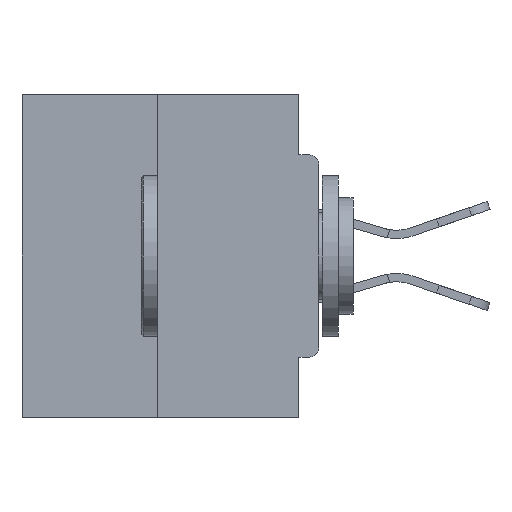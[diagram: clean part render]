
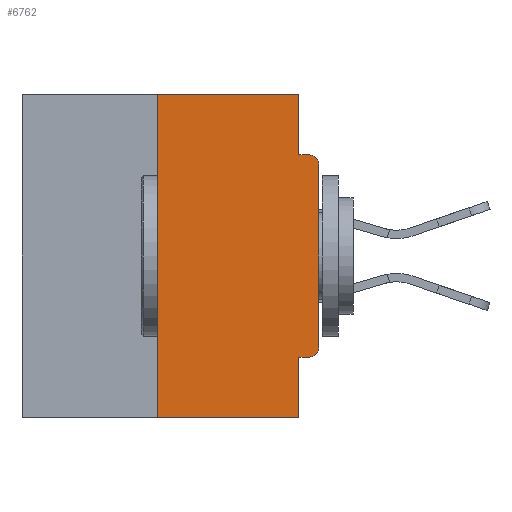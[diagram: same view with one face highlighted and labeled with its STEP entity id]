
A CAD part, left-side view. The second image highlights one B-rep face of the part: STEP entity #6762.
In plain terms, the highlighted planar face has unit normal (-1, 0, 0).
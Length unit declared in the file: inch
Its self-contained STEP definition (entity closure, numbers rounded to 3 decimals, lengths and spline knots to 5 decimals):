
#129 = VERTEX_POINT ( 'NONE', #37225 ) ;
#652 = LINE ( 'NONE', #36962, #32376 ) ;
#769 = ORIENTED_EDGE ( 'NONE', *, *, #18249, .F. ) ;
#838 = DIRECTION ( 'NONE',  ( -1., 0., 0. ) ) ;
#1036 = EDGE_LOOP ( 'NONE', ( #4687, #27229, #32457, #11501, #16882, #5489, #13640, #4862, #15352, #769 ) ) ;
#1515 = EDGE_CURVE ( 'NONE', #34537, #17718, #652, .T. ) ;
#1567 = EDGE_CURVE ( 'NONE', #35840, #129, #34365, .T. ) ;
#3018 = VERTEX_POINT ( 'NONE', #20286 ) ;
#3319 = VERTEX_POINT ( 'NONE', #10467 ) ;
#4687 = ORIENTED_EDGE ( 'NONE', *, *, #25643, .F. ) ;
#4862 = ORIENTED_EDGE ( 'NONE', *, *, #39757, .T. ) ;
#5489 = ORIENTED_EDGE ( 'NONE', *, *, #23468, .T. ) ;
#6762 = ADVANCED_FACE ( 'NONE', ( #23129 ), #31804, .F. ) ;
#7204 = DIRECTION ( 'NONE',  ( 0., 0., -1. ) ) ;
#7487 = LINE ( 'NONE', #32977, #12406 ) ;
#8278 = AXIS2_PLACEMENT_3D ( 'NONE', #34851, #838, #7204 ) ;
#8738 = CARTESIAN_POINT ( 'NONE',  ( 0., 0.031, -0.5 ) ) ;
#8746 = VECTOR ( 'NONE', #33894, 39.37008 ) ;
#9905 = VECTOR ( 'NONE', #30949, 39.37008 ) ;
#10383 = LINE ( 'NONE', #31105, #28981 ) ;
#10467 = CARTESIAN_POINT ( 'NONE',  ( 0., 0.25, -0.5 ) ) ;
#10676 = VERTEX_POINT ( 'NONE', #13329 ) ;
#11501 = ORIENTED_EDGE ( 'NONE', *, *, #18194, .F. ) ;
#11875 = DIRECTION ( 'NONE',  ( 0., 0., -1. ) ) ;
#12406 = VECTOR ( 'NONE', #39248, 39.37008 ) ;
#12536 = DIRECTION ( 'NONE',  ( 0., 0., 1. ) ) ;
#13329 = CARTESIAN_POINT ( 'NONE',  ( 0., 0.031, 0. ) ) ;
#13640 = ORIENTED_EDGE ( 'NONE', *, *, #1567, .T. ) ;
#13912 = EDGE_CURVE ( 'NONE', #3319, #16950, #10383, .T. ) ;
#15352 = ORIENTED_EDGE ( 'NONE', *, *, #1515, .F. ) ;
#15774 = CARTESIAN_POINT ( 'NONE',  ( 0., 0., -0.4065 ) ) ;
#16099 = VECTOR ( 'NONE', #11875, 39.37008 ) ;
#16106 = CARTESIAN_POINT ( 'NONE',  ( 0., 0.46, 0. ) ) ;
#16556 = DIRECTION ( 'NONE',  ( 0., 0., -1. ) ) ;
#16637 = DIRECTION ( 'NONE',  ( 1., 0., 0. ) ) ;
#16882 = ORIENTED_EDGE ( 'NONE', *, *, #21723, .F. ) ;
#16950 = VERTEX_POINT ( 'NONE', #20028 ) ;
#17718 = VERTEX_POINT ( 'NONE', #20878 ) ;
#17770 = CARTESIAN_POINT ( 'NONE',  ( 0., 0.031, -0.4065 ) ) ;
#18194 = EDGE_CURVE ( 'NONE', #32849, #3018, #19501, .T. ) ;
#18249 = EDGE_CURVE ( 'NONE', #10676, #34537, #26800, .T. ) ;
#19450 = CIRCLE ( 'NONE', #30038, 0.015 ) ;
#19501 = LINE ( 'NONE', #8738, #16099 ) ;
#19564 = CARTESIAN_POINT ( 'NONE',  ( 0., 0.015, -0.3915 ) ) ;
#19647 = DIRECTION ( 'NONE',  ( 0., 0., -1. ) ) ;
#20028 = CARTESIAN_POINT ( 'NONE',  ( 0., 0.25, 0. ) ) ;
#20216 = LINE ( 'NONE', #15774, #35386 ) ;
#20286 = CARTESIAN_POINT ( 'NONE',  ( 0., 0.031, -0.5 ) ) ;
#20372 = VECTOR ( 'NONE', #27808, 39.37008 ) ;
#20878 = CARTESIAN_POINT ( 'NONE',  ( 0., 0.015, -0.0935 ) ) ;
#21340 = CARTESIAN_POINT ( 'NONE',  ( 0., 0.031, 0. ) ) ;
#21580 = CARTESIAN_POINT ( 'NONE',  ( 0., 0., -0.3915 ) ) ;
#21723 = EDGE_CURVE ( 'NONE', #25903, #32849, #20216, .T. ) ;
#22712 = DIRECTION ( 'NONE',  ( -1., 0., 0. ) ) ;
#23129 = FACE_OUTER_BOUND ( 'NONE', #1036, .T. ) ;
#23468 = EDGE_CURVE ( 'NONE', #25903, #35840, #19450, .T. ) ;
#24733 = CARTESIAN_POINT ( 'NONE',  ( 0., 0.015, -0.4065 ) ) ;
#25643 = EDGE_CURVE ( 'NONE', #16950, #10676, #7487, .T. ) ;
#25903 = VERTEX_POINT ( 'NONE', #24733 ) ;
#26800 = LINE ( 'NONE', #21340, #8746 ) ;
#27229 = ORIENTED_EDGE ( 'NONE', *, *, #13912, .F. ) ;
#27804 = CARTESIAN_POINT ( 'NONE',  ( 0., 0., 0. ) ) ;
#27808 = DIRECTION ( 'NONE',  ( 0., -1., 0. ) ) ;
#28981 = VECTOR ( 'NONE', #12536, 39.37008 ) ;
#30038 = AXIS2_PLACEMENT_3D ( 'NONE', #19564, #22712, #16556 ) ;
#30139 = CARTESIAN_POINT ( 'NONE',  ( 0., 0.031, -0.0935 ) ) ;
#30523 = CIRCLE ( 'NONE', #8278, 0.015 ) ;
#30545 = EDGE_CURVE ( 'NONE', #3319, #3018, #31626, .T. ) ;
#30583 = AXIS2_PLACEMENT_3D ( 'NONE', #16106, #16637, #19647 ) ;
#30804 = DIRECTION ( 'NONE',  ( 0., -1., 0. ) ) ;
#30949 = DIRECTION ( 'NONE',  ( 0., 0., 1. ) ) ;
#31105 = CARTESIAN_POINT ( 'NONE',  ( 0., 0.25, 0. ) ) ;
#31626 = LINE ( 'NONE', #40239, #20372 ) ;
#31804 = PLANE ( 'NONE',  #30583 ) ;
#32376 = VECTOR ( 'NONE', #30804, 39.37008 ) ;
#32457 = ORIENTED_EDGE ( 'NONE', *, *, #30545, .T. ) ;
#32849 = VERTEX_POINT ( 'NONE', #17770 ) ;
#32977 = CARTESIAN_POINT ( 'NONE',  ( 0., 0.46, 0. ) ) ;
#33894 = DIRECTION ( 'NONE',  ( 0., 0., -1. ) ) ;
#33937 = DIRECTION ( 'NONE',  ( 0., 1., 0. ) ) ;
#34365 = LINE ( 'NONE', #27804, #9905 ) ;
#34537 = VERTEX_POINT ( 'NONE', #30139 ) ;
#34851 = CARTESIAN_POINT ( 'NONE',  ( 0., 0.015, -0.1085 ) ) ;
#35386 = VECTOR ( 'NONE', #33937, 39.37008 ) ;
#35840 = VERTEX_POINT ( 'NONE', #21580 ) ;
#36962 = CARTESIAN_POINT ( 'NONE',  ( 0., 0., -0.0935 ) ) ;
#37225 = CARTESIAN_POINT ( 'NONE',  ( 0., 0., -0.1085 ) ) ;
#39248 = DIRECTION ( 'NONE',  ( 0., -1., 0. ) ) ;
#39757 = EDGE_CURVE ( 'NONE', #129, #17718, #30523, .T. ) ;
#40239 = CARTESIAN_POINT ( 'NONE',  ( 0., 0.46, -0.5 ) ) ;
